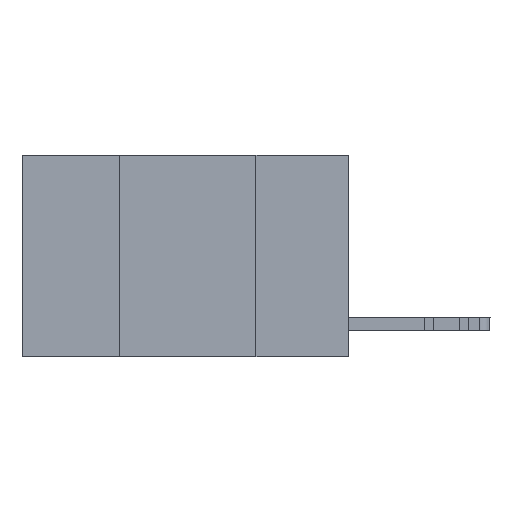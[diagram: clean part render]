
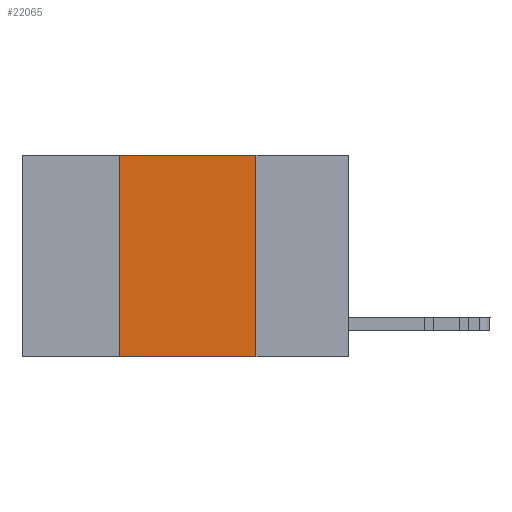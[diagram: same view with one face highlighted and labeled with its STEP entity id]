
A CAD part, left-side view. The second image highlights one B-rep face of the part: STEP entity #22065.
In plain terms, the highlighted planar face has unit normal (-1, 0, 0).
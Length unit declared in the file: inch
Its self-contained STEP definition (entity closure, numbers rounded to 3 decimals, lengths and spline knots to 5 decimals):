
#686 = EDGE_CURVE ( 'NONE', #12929, #23360, #1319, .T. ) ;
#1319 = LINE ( 'NONE', #7415, #18652 ) ;
#1406 = LINE ( 'NONE', #22960, #12877 ) ;
#3157 = LINE ( 'NONE', #16584, #20391 ) ;
#3330 = DIRECTION ( 'NONE',  ( 0., 0., -1. ) ) ;
#5062 = DIRECTION ( 'NONE',  ( 0., -1., 0. ) ) ;
#5184 = VECTOR ( 'NONE', #27073, 39.37008 ) ;
#5530 = FACE_OUTER_BOUND ( 'NONE', #25428, .T. ) ;
#7099 = CARTESIAN_POINT ( 'NONE',  ( 0., 0.17, 0. ) ) ;
#7415 = CARTESIAN_POINT ( 'NONE',  ( 0., 0.42, 0. ) ) ;
#7510 = DIRECTION ( 'NONE',  ( 0., 0., 1. ) ) ;
#9825 = DIRECTION ( 'NONE',  ( 0., -1., 0. ) ) ;
#10088 = PLANE ( 'NONE',  #24885 ) ;
#12877 = VECTOR ( 'NONE', #5062, 39.37008 ) ;
#12929 = VERTEX_POINT ( 'NONE', #24567 ) ;
#15674 = VERTEX_POINT ( 'NONE', #22859 ) ;
#16278 = CARTESIAN_POINT ( 'NONE',  ( 0., 0.17, -0.37 ) ) ;
#16584 = CARTESIAN_POINT ( 'NONE',  ( 0., 0.6, 0. ) ) ;
#16727 = ORIENTED_EDGE ( 'NONE', *, *, #21845, .F. ) ;
#16753 = ORIENTED_EDGE ( 'NONE', *, *, #19396, .F. ) ;
#16838 = DIRECTION ( 'NONE',  ( 1., 0., 0. ) ) ;
#17207 = ORIENTED_EDGE ( 'NONE', *, *, #686, .F. ) ;
#17781 = LINE ( 'NONE', #7099, #5184 ) ;
#18175 = ORIENTED_EDGE ( 'NONE', *, *, #23936, .T. ) ;
#18652 = VECTOR ( 'NONE', #7510, 39.37008 ) ;
#19396 = EDGE_CURVE ( 'NONE', #23360, #15674, #3157, .T. ) ;
#20391 = VECTOR ( 'NONE', #9825, 39.37008 ) ;
#21132 = CARTESIAN_POINT ( 'NONE',  ( 0., 0.42, 0. ) ) ;
#21208 = CARTESIAN_POINT ( 'NONE',  ( 0., 0.6, 0. ) ) ;
#21845 = EDGE_CURVE ( 'NONE', #15674, #25046, #17781, .T. ) ;
#22065 = ADVANCED_FACE ( 'NONE', ( #5530 ), #10088, .F. ) ;
#22859 = CARTESIAN_POINT ( 'NONE',  ( 0., 0.17, 0. ) ) ;
#22960 = CARTESIAN_POINT ( 'NONE',  ( 0., 0.6, -0.37 ) ) ;
#23360 = VERTEX_POINT ( 'NONE', #21132 ) ;
#23936 = EDGE_CURVE ( 'NONE', #12929, #25046, #1406, .T. ) ;
#24567 = CARTESIAN_POINT ( 'NONE',  ( 0., 0.42, -0.37 ) ) ;
#24885 = AXIS2_PLACEMENT_3D ( 'NONE', #21208, #16838, #3330 ) ;
#25046 = VERTEX_POINT ( 'NONE', #16278 ) ;
#25428 = EDGE_LOOP ( 'NONE', ( #16727, #16753, #17207, #18175 ) ) ;
#27073 = DIRECTION ( 'NONE',  ( 0., 0., -1. ) ) ;
